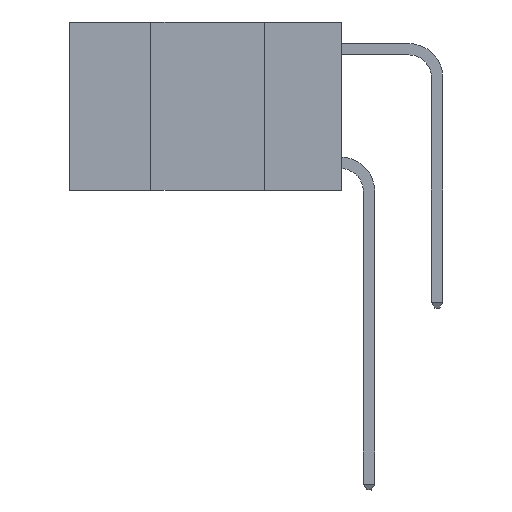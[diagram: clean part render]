
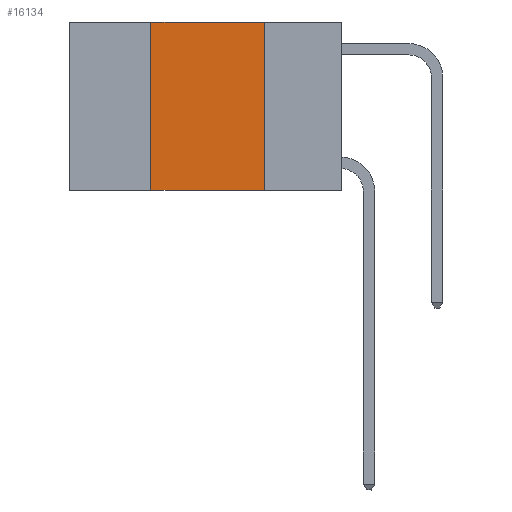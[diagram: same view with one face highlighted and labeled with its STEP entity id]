
A CAD part, left-side view. The second image highlights one B-rep face of the part: STEP entity #16134.
In plain terms, the highlighted planar face has unit normal (-1, 0, 0).
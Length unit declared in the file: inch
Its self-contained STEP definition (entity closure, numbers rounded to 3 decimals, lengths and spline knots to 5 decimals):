
#795 = ORIENTED_EDGE ( 'NONE', *, *, #9081, .F. ) ;
#1176 = CARTESIAN_POINT ( 'NONE',  ( 0., 0.6, 0. ) ) ;
#1437 = CARTESIAN_POINT ( 'NONE',  ( 0., 0.42, -0.37 ) ) ;
#1603 = EDGE_LOOP ( 'NONE', ( #2166, #1653, #795, #9769 ) ) ;
#1653 = ORIENTED_EDGE ( 'NONE', *, *, #5354, .F. ) ;
#1739 = LINE ( 'NONE', #10059, #5115 ) ;
#2166 = ORIENTED_EDGE ( 'NONE', *, *, #14151, .F. ) ;
#2816 = DIRECTION ( 'NONE',  ( 0., 0., -1. ) ) ;
#3975 = VECTOR ( 'NONE', #2816, 39.37008 ) ;
#4255 = PLANE ( 'NONE',  #4703 ) ;
#4267 = DIRECTION ( 'NONE',  ( 0., 0., 1. ) ) ;
#4538 = DIRECTION ( 'NONE',  ( 0., -1., 0. ) ) ;
#4564 = FACE_OUTER_BOUND ( 'NONE', #1603, .T. ) ;
#4703 = AXIS2_PLACEMENT_3D ( 'NONE', #11500, #12952, #17137 ) ;
#4788 = VECTOR ( 'NONE', #4538, 39.37008 ) ;
#5115 = VECTOR ( 'NONE', #4267, 39.37008 ) ;
#5148 = CARTESIAN_POINT ( 'NONE',  ( 0., 0.17, 0. ) ) ;
#5354 = EDGE_CURVE ( 'NONE', #6742, #9444, #7304, .T. ) ;
#6742 = VERTEX_POINT ( 'NONE', #15400 ) ;
#6847 = VECTOR ( 'NONE', #12208, 39.37008 ) ;
#7304 = LINE ( 'NONE', #1176, #4788 ) ;
#9081 = EDGE_CURVE ( 'NONE', #14182, #6742, #1739, .T. ) ;
#9444 = VERTEX_POINT ( 'NONE', #5148 ) ;
#9769 = ORIENTED_EDGE ( 'NONE', *, *, #12536, .T. ) ;
#9832 = LINE ( 'NONE', #18435, #3975 ) ;
#10059 = CARTESIAN_POINT ( 'NONE',  ( 0., 0.42, 0. ) ) ;
#10785 = CARTESIAN_POINT ( 'NONE',  ( 0., 0.17, -0.37 ) ) ;
#11500 = CARTESIAN_POINT ( 'NONE',  ( 0., 0.6, 0. ) ) ;
#11709 = LINE ( 'NONE', #17896, #6847 ) ;
#12208 = DIRECTION ( 'NONE',  ( 0., -1., 0. ) ) ;
#12452 = VERTEX_POINT ( 'NONE', #10785 ) ;
#12536 = EDGE_CURVE ( 'NONE', #14182, #12452, #11709, .T. ) ;
#12952 = DIRECTION ( 'NONE',  ( 1., 0., 0. ) ) ;
#14151 = EDGE_CURVE ( 'NONE', #9444, #12452, #9832, .T. ) ;
#14182 = VERTEX_POINT ( 'NONE', #1437 ) ;
#15400 = CARTESIAN_POINT ( 'NONE',  ( 0., 0.42, 0. ) ) ;
#16134 = ADVANCED_FACE ( 'NONE', ( #4564 ), #4255, .F. ) ;
#17137 = DIRECTION ( 'NONE',  ( 0., 0., -1. ) ) ;
#17896 = CARTESIAN_POINT ( 'NONE',  ( 0., 0.6, -0.37 ) ) ;
#18435 = CARTESIAN_POINT ( 'NONE',  ( 0., 0.17, 0. ) ) ;
